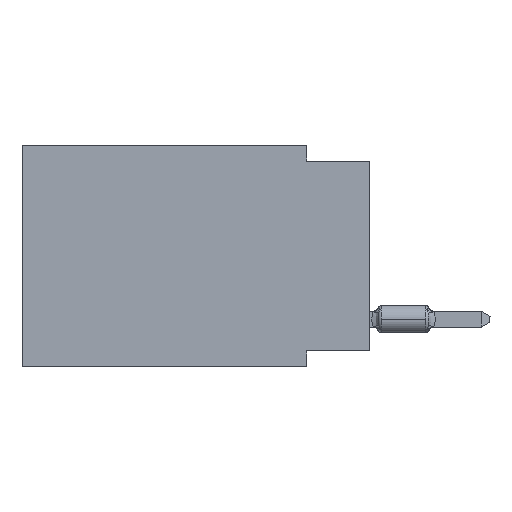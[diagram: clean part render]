
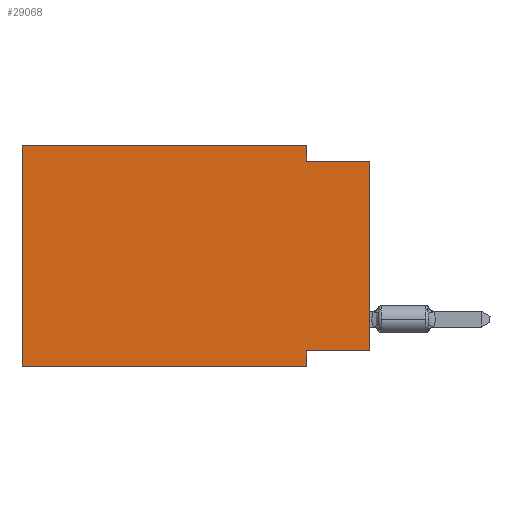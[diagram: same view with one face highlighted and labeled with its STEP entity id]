
A CAD part, left-side view. The second image highlights one B-rep face of the part: STEP entity #29068.
In plain terms, the highlighted planar face has unit normal (-1, 0, 0).
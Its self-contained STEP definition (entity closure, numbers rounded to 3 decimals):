
#1057 = CARTESIAN_POINT ( 'NONE',  ( 0., 2.54, -8.255 ) ) ;
#1334 = VERTEX_POINT ( 'NONE', #44856 ) ;
#1424 = EDGE_CURVE ( 'NONE', #29022, #32439, #34650, .T. ) ;
#1592 = AXIS2_PLACEMENT_3D ( 'NONE', #41940, #34643, #34889 ) ;
#1775 = LINE ( 'NONE', #5416, #20004 ) ;
#2060 = DIRECTION ( 'NONE',  ( 0., 0., 1. ) ) ;
#2338 = CARTESIAN_POINT ( 'NONE',  ( 0., 13.97, 0. ) ) ;
#4182 = LINE ( 'NONE', #34595, #34016 ) ;
#4986 = CARTESIAN_POINT ( 'NONE',  ( 0., 0., 0. ) ) ;
#5326 = DIRECTION ( 'NONE',  ( 0., -1., 0. ) ) ;
#5416 = CARTESIAN_POINT ( 'NONE',  ( 0., 2.54, 0. ) ) ;
#5881 = CARTESIAN_POINT ( 'NONE',  ( 0., 2.54, -8.89 ) ) ;
#6161 = CARTESIAN_POINT ( 'NONE',  ( 0., 13.97, 0. ) ) ;
#6614 = ORIENTED_EDGE ( 'NONE', *, *, #27473, .T. ) ;
#8818 = VERTEX_POINT ( 'NONE', #25618 ) ;
#8980 = ORIENTED_EDGE ( 'NONE', *, *, #1424, .F. ) ;
#9952 = VECTOR ( 'NONE', #5326, 1000. ) ;
#10180 = CARTESIAN_POINT ( 'NONE',  ( 0., 0., -0.635 ) ) ;
#11170 = EDGE_LOOP ( 'NONE', ( #35220, #39167, #47702, #38873, #26815, #6614, #8980, #29525 ) ) ;
#11794 = FACE_OUTER_BOUND ( 'NONE', #11170, .T. ) ;
#14599 = CARTESIAN_POINT ( 'NONE',  ( 0., 0., -8.255 ) ) ;
#16078 = CARTESIAN_POINT ( 'NONE',  ( 0., 2.54, 0. ) ) ;
#17669 = LINE ( 'NONE', #2338, #48146 ) ;
#18650 = LINE ( 'NONE', #33493, #36426 ) ;
#19362 = DIRECTION ( 'NONE',  ( 0., -1., 0. ) ) ;
#20004 = VECTOR ( 'NONE', #28053, 1000. ) ;
#20580 = LINE ( 'NONE', #4986, #29262 ) ;
#21449 = VERTEX_POINT ( 'NONE', #6161 ) ;
#21831 = EDGE_CURVE ( 'NONE', #36299, #42764, #4182, .T. ) ;
#23758 = EDGE_CURVE ( 'NONE', #21449, #26626, #45968, .T. ) ;
#25618 = CARTESIAN_POINT ( 'NONE',  ( 0., 13.97, -8.89 ) ) ;
#26271 = EDGE_CURVE ( 'NONE', #26626, #36299, #1775, .T. ) ;
#26626 = VERTEX_POINT ( 'NONE', #16078 ) ;
#26815 = ORIENTED_EDGE ( 'NONE', *, *, #43607, .F. ) ;
#27107 = PLANE ( 'NONE',  #1592 ) ;
#27116 = DIRECTION ( 'NONE',  ( 0., 0., -1. ) ) ;
#27473 = EDGE_CURVE ( 'NONE', #8818, #32439, #18650, .T. ) ;
#27668 = DIRECTION ( 'NONE',  ( 0., 0., 1. ) ) ;
#27966 = CARTESIAN_POINT ( 'NONE',  ( 0., 13.97, 0. ) ) ;
#28053 = DIRECTION ( 'NONE',  ( 0., 0., -1. ) ) ;
#29022 = VERTEX_POINT ( 'NONE', #1057 ) ;
#29068 = ADVANCED_FACE ( 'NONE', ( #11794 ), #27107, .F. ) ;
#29262 = VECTOR ( 'NONE', #2060, 1000. ) ;
#29525 = ORIENTED_EDGE ( 'NONE', *, *, #42466, .F. ) ;
#32439 = VERTEX_POINT ( 'NONE', #5881 ) ;
#33079 = LINE ( 'NONE', #14599, #40320 ) ;
#33493 = CARTESIAN_POINT ( 'NONE',  ( 0., 13.97, -8.89 ) ) ;
#34016 = VECTOR ( 'NONE', #41159, 1000. ) ;
#34595 = CARTESIAN_POINT ( 'NONE',  ( 0., 0., -0.635 ) ) ;
#34643 = DIRECTION ( 'NONE',  ( 1., 0., 0. ) ) ;
#34650 = LINE ( 'NONE', #34900, #37617 ) ;
#34889 = DIRECTION ( 'NONE',  ( 0., 0., -1. ) ) ;
#34900 = CARTESIAN_POINT ( 'NONE',  ( 0., 2.54, -8.89 ) ) ;
#35220 = ORIENTED_EDGE ( 'NONE', *, *, #39260, .T. ) ;
#36299 = VERTEX_POINT ( 'NONE', #37372 ) ;
#36426 = VECTOR ( 'NONE', #19362, 1000. ) ;
#37372 = CARTESIAN_POINT ( 'NONE',  ( 0., 2.54, -0.635 ) ) ;
#37433 = DIRECTION ( 'NONE',  ( 0., 1., 0. ) ) ;
#37617 = VECTOR ( 'NONE', #27116, 1000. ) ;
#38873 = ORIENTED_EDGE ( 'NONE', *, *, #23758, .F. ) ;
#39167 = ORIENTED_EDGE ( 'NONE', *, *, #21831, .F. ) ;
#39260 = EDGE_CURVE ( 'NONE', #1334, #42764, #20580, .T. ) ;
#40320 = VECTOR ( 'NONE', #37433, 1000. ) ;
#41159 = DIRECTION ( 'NONE',  ( 0., -1., 0. ) ) ;
#41940 = CARTESIAN_POINT ( 'NONE',  ( 0., 13.97, 0. ) ) ;
#42466 = EDGE_CURVE ( 'NONE', #1334, #29022, #33079, .T. ) ;
#42764 = VERTEX_POINT ( 'NONE', #10180 ) ;
#43607 = EDGE_CURVE ( 'NONE', #8818, #21449, #17669, .T. ) ;
#44856 = CARTESIAN_POINT ( 'NONE',  ( 0., 0., -8.255 ) ) ;
#45968 = LINE ( 'NONE', #27966, #9952 ) ;
#47702 = ORIENTED_EDGE ( 'NONE', *, *, #26271, .F. ) ;
#48146 = VECTOR ( 'NONE', #27668, 1000. ) ;
